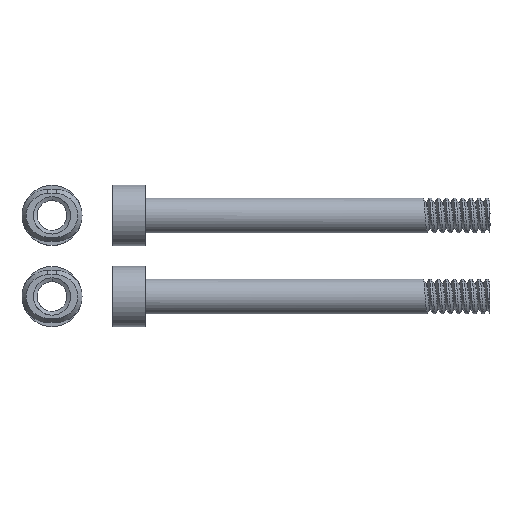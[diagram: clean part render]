
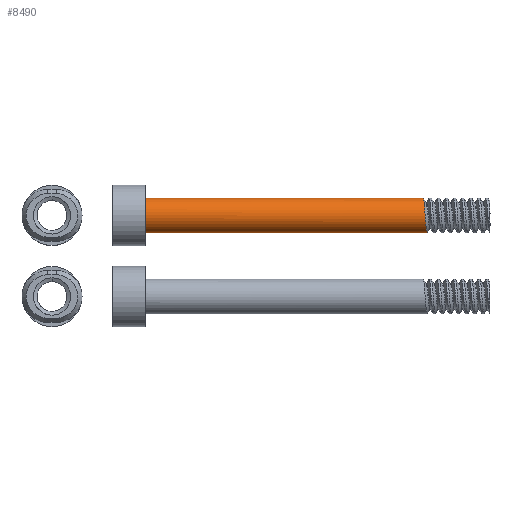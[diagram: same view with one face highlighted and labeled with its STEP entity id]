
A CAD part, top view. The second image highlights one B-rep face of the part: STEP entity #8490.
In plain terms, the highlighted cylindrical face has radius 2.731 mm (diameter 5.461 mm), a partial arc.
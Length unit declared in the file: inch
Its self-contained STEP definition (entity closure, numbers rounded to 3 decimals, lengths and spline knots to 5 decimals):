
#70 = CARTESIAN_POINT ( 'NONE',  ( -0.19831, 0.26516, 1.90153 ) ) ;
#341 = ORIENTED_EDGE ( 'NONE', *, *, #2816, .T. ) ;
#578 = ORIENTED_EDGE ( 'NONE', *, *, #993, .T. ) ;
#602 = DIRECTION ( 'NONE',  ( 0., -1., 0. ) ) ;
#993 = EDGE_CURVE ( 'NONE', #9023, #8381, #3537, .T. ) ;
#1149 = CARTESIAN_POINT ( 'NONE',  ( -0.19831, 0.48016, 1.90153 ) ) ;
#1322 = EDGE_CURVE ( 'NONE', #8738, #8737, #1718, .T. ) ;
#1332 = CARTESIAN_POINT ( 'NONE',  ( -0.19831, 0.37266, 1.90153 ) ) ;
#1718 = CIRCLE ( 'NONE', #5410, 0.1075 ) ;
#1906 = LINE ( 'NONE', #2955, #3188 ) ;
#1922 = LINE ( 'NONE', #6461, #6828 ) ;
#2149 = AXIS2_PLACEMENT_3D ( 'NONE', #6552, #5287, #9007 ) ;
#2400 = CARTESIAN_POINT ( 'NONE',  ( 1.52044, 0.44868, 1.97754 ) ) ;
#2816 = EDGE_CURVE ( 'NONE', #8381, #6089, #8499, .T. ) ;
#2955 = CARTESIAN_POINT ( 'NONE',  ( -0.19831, 0.26516, 1.90153 ) ) ;
#3025 = CARTESIAN_POINT ( 'NONE',  ( 1.52357, 0.41719, 2.00903 ) ) ;
#3043 = VERTEX_POINT ( 'NONE', #7997 ) ;
#3116 = CARTESIAN_POINT ( 'NONE',  ( 1.52982, 0.32814, 2.00903 ) ) ;
#3188 = VECTOR ( 'NONE', #8162, 39.37008 ) ;
#3525 = CARTESIAN_POINT ( 'NONE',  ( -0.19831, 0.26516, 1.90153 ) ) ;
#3537 = LINE ( 'NONE', #70, #5279 ) ;
#3867 = ORIENTED_EDGE ( 'NONE', *, *, #6179, .F. ) ;
#4239 = CYLINDRICAL_SURFACE ( 'NONE', #2149, 0.1075 ) ;
#4503 = DIRECTION ( 'NONE',  ( 1., 0., 0. ) ) ;
#5240 = ORIENTED_EDGE ( 'NONE', *, *, #6383, .F. ) ;
#5279 = VECTOR ( 'NONE', #4503, 39.37008 ) ;
#5287 = DIRECTION ( 'NONE',  ( 1., 0., 0. ) ) ;
#5394 = FACE_OUTER_BOUND ( 'NONE', #6212, .T. ) ;
#5410 = AXIS2_PLACEMENT_3D ( 'NONE', #1332, #7234, #602 ) ;
#5863 = CARTESIAN_POINT ( 'NONE',  ( 1.52669, 0.26516, 1.90153 ) ) ;
#5865 = ORIENTED_EDGE ( 'NONE', *, *, #9409, .T. ) ;
#6087 = CARTESIAN_POINT ( 'NONE',  ( 1.53607, 0.26516, 1.94606 ) ) ;
#6089 = VERTEX_POINT ( 'NONE', #9135 ) ;
#6130 = CARTESIAN_POINT ( 'NONE',  ( 1.50794, 0.26516, 1.90153 ) ) ;
#6179 = EDGE_CURVE ( 'NONE', #9023, #3043, #8218, .T. ) ;
#6212 = EDGE_LOOP ( 'NONE', ( #8164, #5865, #3867, #578, #341, #5240 ) ) ;
#6383 = EDGE_CURVE ( 'NONE', #8737, #6089, #1922, .T. ) ;
#6461 = CARTESIAN_POINT ( 'NONE',  ( -0.19831, 0.48016, 1.90153 ) ) ;
#6552 = CARTESIAN_POINT ( 'NONE',  ( -0.19831, 0.37266, 1.90153 ) ) ;
#6828 = VECTOR ( 'NONE', #8808, 39.37008 ) ;
#6851 = DIRECTION ( 'NONE',  ( -1., 0., 0. ) ) ;
#7234 = DIRECTION ( 'NONE',  ( -1., 0., 0. ) ) ;
#7580 = CARTESIAN_POINT ( 'NONE',  ( 1.53294, 0.29665, 1.97754 ) ) ;
#7997 = CARTESIAN_POINT ( 'NONE',  ( 1.48919, 0.26516, 1.90153 ) ) ;
#8162 = DIRECTION ( 'NONE',  ( 1., 0., 0. ) ) ;
#8164 = ORIENTED_EDGE ( 'NONE', *, *, #1322, .F. ) ;
#8218 = LINE ( 'NONE', #6130, #8691 ) ;
#8269 = CARTESIAN_POINT ( 'NONE',  ( 1.53919, 0.26516, 1.90153 ) ) ;
#8340 = CARTESIAN_POINT ( 'NONE',  ( 1.52669, 0.37266, 2.00903 ) ) ;
#8368 = CARTESIAN_POINT ( 'NONE',  ( 1.51732, 0.48016, 1.94606 ) ) ;
#8381 = VERTEX_POINT ( 'NONE', #8845 ) ;
#8490 = ADVANCED_FACE ( 'NONE', ( #5394 ), #4239, .T. ) ;
#8499 =( BOUNDED_CURVE ( )  B_SPLINE_CURVE ( 2, ( #8269, #6087, #7580, #3116, #8340, #3025, #2400, #8368, #9685 ),
 .UNSPECIFIED., .F., .T. ) 
 B_SPLINE_CURVE_WITH_KNOTS ( ( 3, 2, 2, 2, 3 ),
 ( 0.88889, 0.90278, 0.91667, 0.93056, 0.94444 ),
 .UNSPECIFIED. ) 
 CURVE ( )  GEOMETRIC_REPRESENTATION_ITEM ( )  RATIONAL_B_SPLINE_CURVE ( ( 1., 0.924, 1., 0.924, 1., 0.924, 1., 0.924, 1. ) ) 
 REPRESENTATION_ITEM ( '' )  );
#8691 = VECTOR ( 'NONE', #6851, 39.37008 ) ;
#8737 = VERTEX_POINT ( 'NONE', #1149 ) ;
#8738 = VERTEX_POINT ( 'NONE', #3525 ) ;
#8808 = DIRECTION ( 'NONE',  ( 1., 0., 0. ) ) ;
#8845 = CARTESIAN_POINT ( 'NONE',  ( 1.53919, 0.26516, 1.90153 ) ) ;
#9007 = DIRECTION ( 'NONE',  ( 0., 1., 0. ) ) ;
#9023 = VERTEX_POINT ( 'NONE', #5863 ) ;
#9135 = CARTESIAN_POINT ( 'NONE',  ( 1.51419, 0.48016, 1.90153 ) ) ;
#9409 = EDGE_CURVE ( 'NONE', #8738, #3043, #1906, .T. ) ;
#9685 = CARTESIAN_POINT ( 'NONE',  ( 1.51419, 0.48016, 1.90153 ) ) ;
